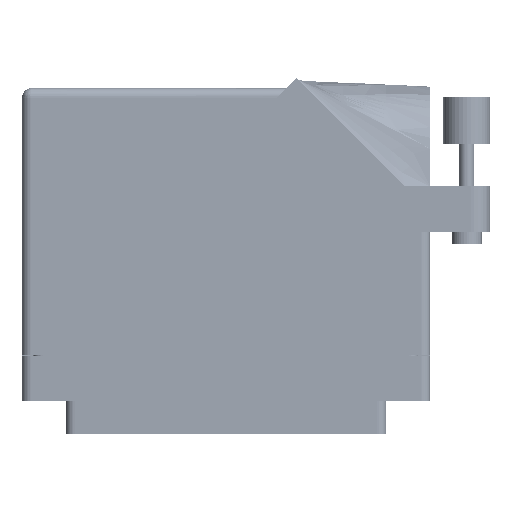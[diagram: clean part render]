
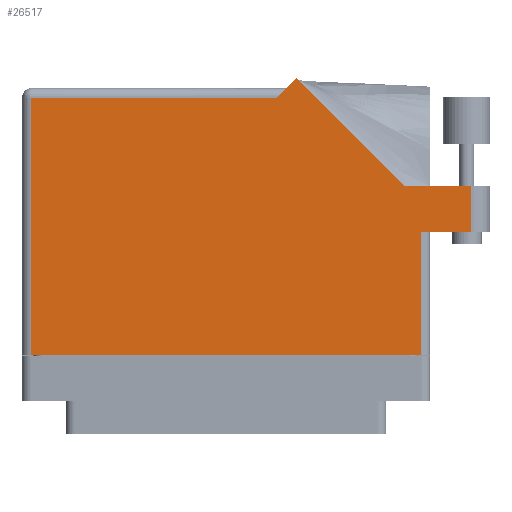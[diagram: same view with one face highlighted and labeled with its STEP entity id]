
A CAD part, front view. The second image highlights one B-rep face of the part: STEP entity #26517.
In plain terms, the highlighted face is planar.
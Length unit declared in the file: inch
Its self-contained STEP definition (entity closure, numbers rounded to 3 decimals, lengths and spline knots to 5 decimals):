
#947 = CARTESIAN_POINT ( 'NONE',  ( 0.46971, 1.74571, 0.617 ) ) ;
#1688 = FACE_OUTER_BOUND ( 'NONE', #72981, .T. ) ;
#1791 = ORIENTED_EDGE ( 'NONE', *, *, #27440, .T. ) ;
#2691 = DIRECTION ( 'NONE',  ( 0., 1., 0. ) ) ;
#3772 = CARTESIAN_POINT ( 'NONE',  ( 1.297, -0.1, 0.617 ) ) ;
#5685 = AXIS2_PLACEMENT_3D ( 'NONE', #70116, #13280, #36089 ) ;
#6834 = VERTEX_POINT ( 'NONE', #63048 ) ;
#7032 = DIRECTION ( 'NONE',  ( 0., 1., 0. ) ) ;
#7590 = CARTESIAN_POINT ( 'NONE',  ( 1.19342, 1.022, 0.617 ) ) ;
#8812 = VECTOR ( 'NONE', #37460, 39.37008 ) ;
#9249 = DIRECTION ( 'NONE',  ( -0.707, 0.707, 0. ) ) ;
#13280 = DIRECTION ( 'NONE',  ( 0., 0., -1. ) ) ;
#15873 = VECTOR ( 'NONE', #9249, 39.37008 ) ;
#18186 = VECTOR ( 'NONE', #40696, 39.37008 ) ;
#18432 = EDGE_CURVE ( 'NONE', #44313, #35007, #51898, .T. ) ;
#18450 = EDGE_CURVE ( 'NONE', #18755, #39479, #69837, .T. ) ;
#18609 = CARTESIAN_POINT ( 'NONE',  ( 1.634, 1.022, 0.617 ) ) ;
#18755 = VERTEX_POINT ( 'NONE', #43988 ) ;
#19699 = CARTESIAN_POINT ( 'NONE',  ( -1.297, 1.613, 0.617 ) ) ;
#24212 = DIRECTION ( 'NONE',  ( -0.707, -0.707, 0. ) ) ;
#24483 = PLANE ( 'NONE',  #5685 ) ;
#26517 = ADVANCED_FACE ( 'NONE', ( #1688 ), #24483, .F. ) ;
#27440 = EDGE_CURVE ( 'NONE', #6834, #68376, #38396, .T. ) ;
#29468 = CARTESIAN_POINT ( 'NONE',  ( -1.359, 1.613, 0.617 ) ) ;
#30571 = LINE ( 'NONE', #29468, #18186 ) ;
#31084 = LINE ( 'NONE', #63003, #51743 ) ;
#31236 = ORIENTED_EDGE ( 'NONE', *, *, #18450, .T. ) ;
#32388 = CARTESIAN_POINT ( 'NONE',  ( 1.19342, 1.022, 0.617 ) ) ;
#32617 = LINE ( 'NONE', #49084, #69945 ) ;
#33024 = VECTOR ( 'NONE', #7032, 39.37008 ) ;
#33508 = CARTESIAN_POINT ( 'NONE',  ( -1.359, -0.1, 0.617 ) ) ;
#34432 = ORIENTED_EDGE ( 'NONE', *, *, #49462, .T. ) ;
#35007 = VERTEX_POINT ( 'NONE', #72500 ) ;
#35422 = CARTESIAN_POINT ( 'NONE',  ( 1.634, 1.022, 0.617 ) ) ;
#36089 = DIRECTION ( 'NONE',  ( -1., 0., 0. ) ) ;
#37460 = DIRECTION ( 'NONE',  ( 0., -1., 0. ) ) ;
#37996 = EDGE_CURVE ( 'NONE', #38484, #18755, #66234, .T. ) ;
#38396 = LINE ( 'NONE', #33508, #49818 ) ;
#38484 = VERTEX_POINT ( 'NONE', #49296 ) ;
#38552 = LINE ( 'NONE', #49763, #8812 ) ;
#38695 = EDGE_CURVE ( 'NONE', #68376, #38484, #31084, .T. ) ;
#38797 = EDGE_CURVE ( 'NONE', #54027, #6834, #38552, .T. ) ;
#39479 = VERTEX_POINT ( 'NONE', #35422 ) ;
#39679 = EDGE_CURVE ( 'NONE', #72618, #44313, #48855, .T. ) ;
#39684 = VECTOR ( 'NONE', #55371, 39.37008 ) ;
#40696 = DIRECTION ( 'NONE',  ( -1., 0., 0. ) ) ;
#42995 = ORIENTED_EDGE ( 'NONE', *, *, #39679, .T. ) ;
#43988 = CARTESIAN_POINT ( 'NONE',  ( 1.634, 0.715, 0.617 ) ) ;
#44313 = VERTEX_POINT ( 'NONE', #947 ) ;
#46357 = ORIENTED_EDGE ( 'NONE', *, *, #66341, .T. ) ;
#46464 = ORIENTED_EDGE ( 'NONE', *, *, #18432, .T. ) ;
#48265 = ORIENTED_EDGE ( 'NONE', *, *, #38797, .T. ) ;
#48855 = LINE ( 'NONE', #32388, #15873 ) ;
#49084 = CARTESIAN_POINT ( 'NONE',  ( 1.759, 1.022, 0.617 ) ) ;
#49296 = CARTESIAN_POINT ( 'NONE',  ( 1.297, 0.715, 0.617 ) ) ;
#49462 = EDGE_CURVE ( 'NONE', #39479, #72618, #32617, .T. ) ;
#49763 = CARTESIAN_POINT ( 'NONE',  ( -1.297, -0.1, 0.617 ) ) ;
#49818 = VECTOR ( 'NONE', #55589, 39.37008 ) ;
#51743 = VECTOR ( 'NONE', #2691, 39.37008 ) ;
#51898 = LINE ( 'NONE', #63479, #58054 ) ;
#54027 = VERTEX_POINT ( 'NONE', #19699 ) ;
#55371 = DIRECTION ( 'NONE',  ( 1., 0., 0. ) ) ;
#55589 = DIRECTION ( 'NONE',  ( 1., 0., 0. ) ) ;
#55736 = CARTESIAN_POINT ( 'NONE',  ( 1.359, 0.715, 0.617 ) ) ;
#58054 = VECTOR ( 'NONE', #24212, 39.37008 ) ;
#61313 = ORIENTED_EDGE ( 'NONE', *, *, #38695, .T. ) ;
#63003 = CARTESIAN_POINT ( 'NONE',  ( 1.297, 0.715, 0.617 ) ) ;
#63048 = CARTESIAN_POINT ( 'NONE',  ( -1.297, -0.1, 0.617 ) ) ;
#63479 = CARTESIAN_POINT ( 'NONE',  ( 0.399, 1.675, 0.617 ) ) ;
#66234 = LINE ( 'NONE', #55736, #39684 ) ;
#66293 = DIRECTION ( 'NONE',  ( -1., 0., 0. ) ) ;
#66341 = EDGE_CURVE ( 'NONE', #35007, #54027, #30571, .T. ) ;
#68376 = VERTEX_POINT ( 'NONE', #3772 ) ;
#69837 = LINE ( 'NONE', #18609, #33024 ) ;
#69945 = VECTOR ( 'NONE', #66293, 39.37008 ) ;
#70116 = CARTESIAN_POINT ( 'NONE',  ( -1.359, 1.675, 0.617 ) ) ;
#71697 = ORIENTED_EDGE ( 'NONE', *, *, #37996, .T. ) ;
#72500 = CARTESIAN_POINT ( 'NONE',  ( 0.337, 1.613, 0.617 ) ) ;
#72618 = VERTEX_POINT ( 'NONE', #7590 ) ;
#72981 = EDGE_LOOP ( 'NONE', ( #71697, #31236, #34432, #42995, #46464, #46357, #48265, #1791, #61313 ) ) ;
